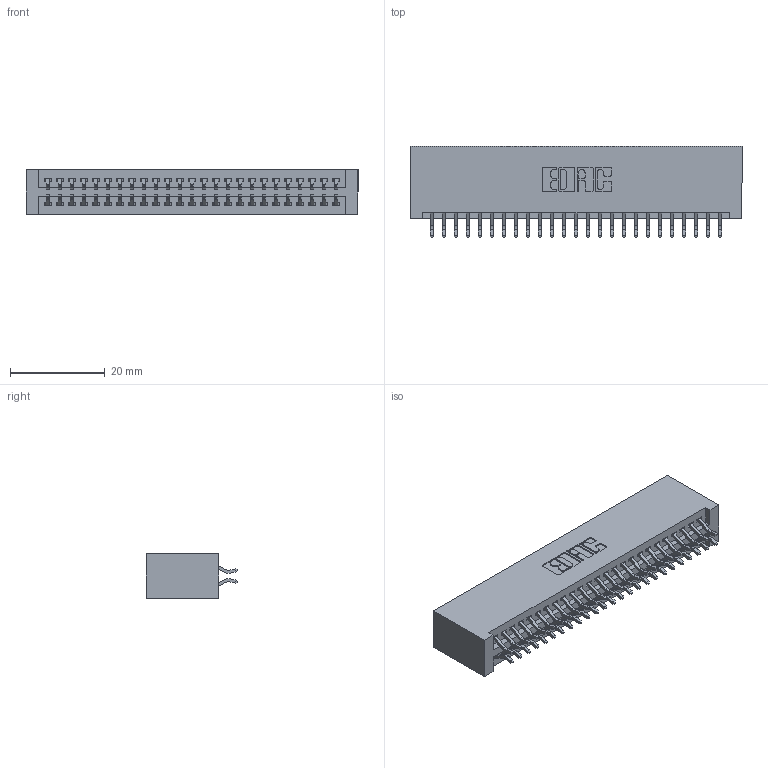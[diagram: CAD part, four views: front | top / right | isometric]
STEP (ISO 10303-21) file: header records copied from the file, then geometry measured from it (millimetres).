
FILE_DESCRIPTION (( 'STEP AP203' ), '1' );
FILE_NAME ('395-050-556-201.STEP', '2018-11-20T10:00:24', ( '' ), ( '' ), 'SwSTEP 2.0', 'SolidWorks 2016', '' );
FILE_SCHEMA (( 'CONFIG_CONTROL_DESIGN' ));
Length unit declared in the file: inch
Products named in the file (3): 395-050-556-201; 345 Part_No Mounting Lugs; 345-292-001_556 Tail
Assembly tree (51 placements, depth 2):
  395-050-556-201
    345 Part_No Mounting Lugs
    345-292-001_556 Tail  x50
Bounding box: 70.1 x 19.24 x 9.4 mm (x, y, z)
Volume: 7266.1 mm3; surface area: 10670.8 mm2
Topology: 51 solids, 51 shells, 2918 faces, 8667 edges, 5710 vertices
Faces by surface type: plane 1926, cylinder 992
Entity records: 21847 total; most frequent: CARTESIAN_POINT 3692, ORIENTED_EDGE 3614, DIRECTION 3259, EDGE_CURVE 1807, VECTOR 1575, LINE 1575, VERTEX_POINT 1202, AXIS2_PLACEMENT_3D 842
